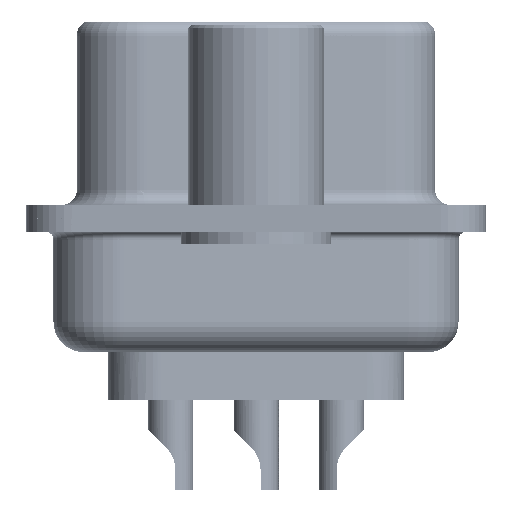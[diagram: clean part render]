
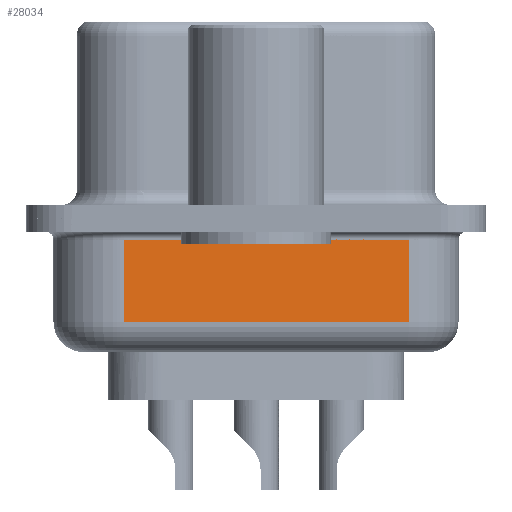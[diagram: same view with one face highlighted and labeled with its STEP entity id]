
A CAD part, left-side view. The second image highlights one B-rep face of the part: STEP entity #28034.
In plain terms, the highlighted planar face has unit normal (-0.985, -0.174, 0).
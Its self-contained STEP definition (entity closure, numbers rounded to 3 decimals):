
#446 = CARTESIAN_POINT ( 'NONE',  ( 2.93, 4.403, -0.7 ) ) ;
#930 = DIRECTION ( 'NONE',  ( 0.174, -0.985, 0. ) ) ;
#967 = CARTESIAN_POINT ( 'NONE',  ( 4.605, -5.097, -0.7 ) ) ;
#1200 = PLANE ( 'NONE',  #26185 ) ;
#1595 = VECTOR ( 'NONE', #27492, 1000. ) ;
#1944 = LINE ( 'NONE', #17503, #13143 ) ;
#2026 = EDGE_CURVE ( 'NONE', #17579, #27214, #20118, .T. ) ;
#2821 = ORIENTED_EDGE ( 'NONE', *, *, #29423, .T. ) ;
#4199 = DIRECTION ( 'NONE',  ( 0.985, 0.174, 0. ) ) ;
#5584 = CARTESIAN_POINT ( 'NONE',  ( 2.93, 4.403, -3.45 ) ) ;
#7031 = FACE_OUTER_BOUND ( 'NONE', #27234, .T. ) ;
#8727 = VECTOR ( 'NONE', #9044, 1000. ) ;
#9044 = DIRECTION ( 'NONE',  ( -0.174, 0.985, 0. ) ) ;
#13143 = VECTOR ( 'NONE', #32435, 1000. ) ;
#14089 = LINE ( 'NONE', #24461, #8727 ) ;
#14573 = CARTESIAN_POINT ( 'NONE',  ( 2.93, 4.403, -4.45 ) ) ;
#14650 = CARTESIAN_POINT ( 'NONE',  ( 4.605, -5.097, -3.45 ) ) ;
#15268 = ORIENTED_EDGE ( 'NONE', *, *, #21961, .T. ) ;
#16415 = VERTEX_POINT ( 'NONE', #446 ) ;
#17262 = CARTESIAN_POINT ( 'NONE',  ( 4.605, -5.097, -4.45 ) ) ;
#17503 = CARTESIAN_POINT ( 'NONE',  ( 2.93, 4.403, -4.45 ) ) ;
#17579 = VERTEX_POINT ( 'NONE', #14650 ) ;
#20118 = LINE ( 'NONE', #17262, #1595 ) ;
#20392 = ORIENTED_EDGE ( 'NONE', *, *, #2026, .T. ) ;
#21961 = EDGE_CURVE ( 'NONE', #27214, #16415, #14089, .T. ) ;
#22265 = DIRECTION ( 'NONE',  ( -0.174, 0.985, 0. ) ) ;
#23120 = EDGE_CURVE ( 'NONE', #27923, #16415, #1944, .T. ) ;
#23856 = CARTESIAN_POINT ( 'NONE',  ( 2.93, 4.403, -3.45 ) ) ;
#24186 = LINE ( 'NONE', #23856, #29934 ) ;
#24461 = CARTESIAN_POINT ( 'NONE',  ( 2.93, 4.403, -0.7 ) ) ;
#26185 = AXIS2_PLACEMENT_3D ( 'NONE', #14573, #4199, #22265 ) ;
#27214 = VERTEX_POINT ( 'NONE', #967 ) ;
#27234 = EDGE_LOOP ( 'NONE', ( #31089, #2821, #20392, #15268 ) ) ;
#27492 = DIRECTION ( 'NONE',  ( 0., 0., 1. ) ) ;
#27923 = VERTEX_POINT ( 'NONE', #5584 ) ;
#28034 = ADVANCED_FACE ( 'NONE', ( #7031 ), #1200, .F. ) ;
#29423 = EDGE_CURVE ( 'NONE', #27923, #17579, #24186, .T. ) ;
#29934 = VECTOR ( 'NONE', #930, 1000. ) ;
#31089 = ORIENTED_EDGE ( 'NONE', *, *, #23120, .F. ) ;
#32435 = DIRECTION ( 'NONE',  ( 0., 0., 1. ) ) ;
